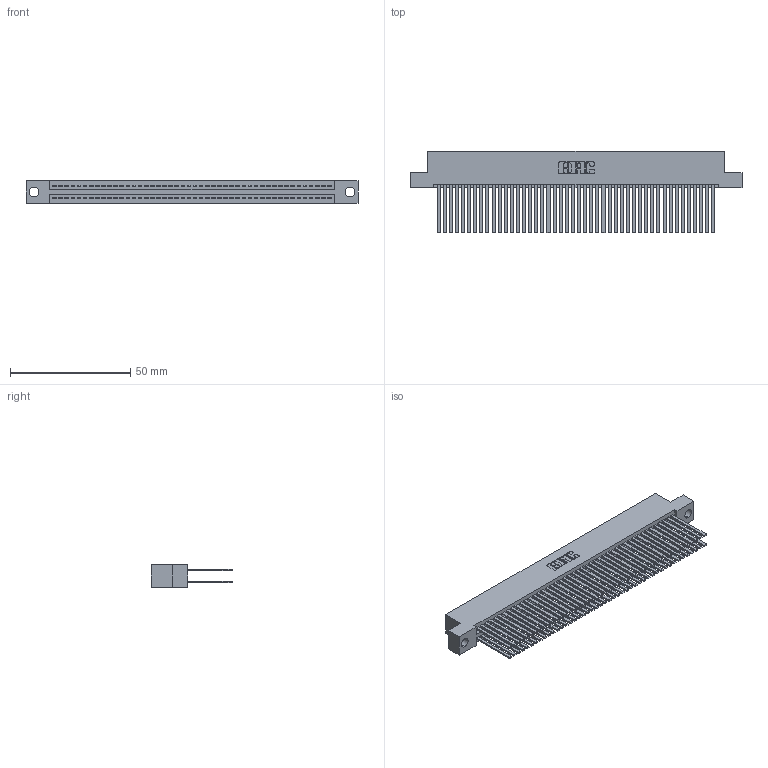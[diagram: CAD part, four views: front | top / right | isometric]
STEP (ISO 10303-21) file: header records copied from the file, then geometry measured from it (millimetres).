
FILE_DESCRIPTION (( 'STEP AP203' ), '1' );
FILE_NAME ('345-092-544-204.STEP', '2021-05-20T15:44:36', ( '' ), ( '' ), 'SwSTEP 2.0', 'SolidWorks 2020', '' );
FILE_SCHEMA (( 'CONFIG_CONTROL_DESIGN' ));
Length unit declared in the file: inch
Products named in the file (3): 345-092-544-204; 345 Part_Flush Mounting Lugs - 0.156 Dia-TI; 345-292-001_345-293-144
Assembly tree (93 placements, depth 2):
  345-092-544-204
    345 Part_Flush Mounting Lugs - 0.156 Dia-TI
    345-292-001_345-293-144  x92
Bounding box: 138.05 x 33.96 x 9.4 mm (x, y, z)
Volume: 14631.1 mm3; surface area: 25336.2 mm2
Topology: 93 solids, 93 shells, 4188 faces, 12429 edges, 8162 vertices
Faces by surface type: plane 2762, cylinder 1426
Entity records: 35789 total; most frequent: CARTESIAN_POINT 5998, ORIENTED_EDGE 5930, DIRECTION 5281, EDGE_CURVE 2965, LINE 2653, VECTOR 2653, VERTEX_POINT 1974, AXIS2_PLACEMENT_3D 1314
